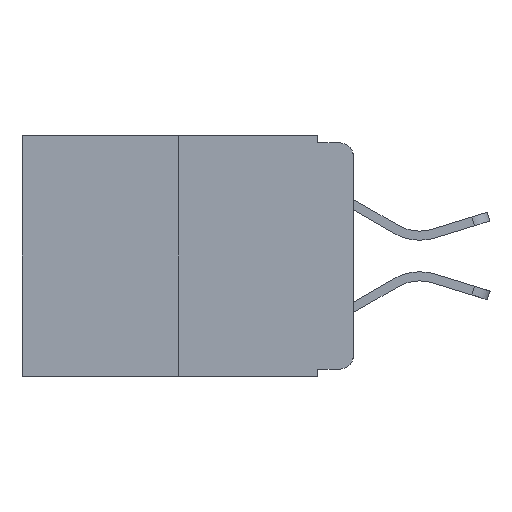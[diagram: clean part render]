
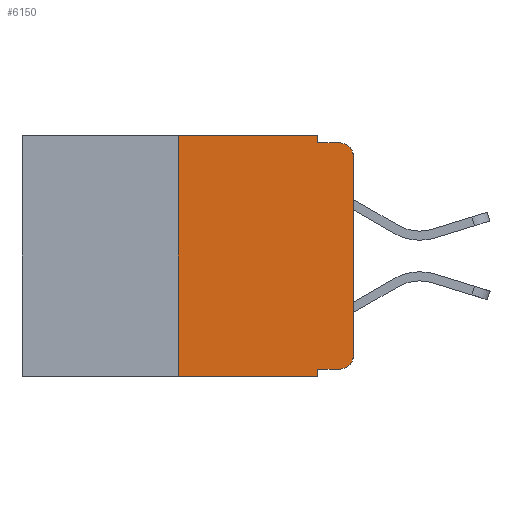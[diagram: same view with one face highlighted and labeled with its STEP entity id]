
A CAD part, left-side view. The second image highlights one B-rep face of the part: STEP entity #6150.
In plain terms, the highlighted planar face has unit normal (-1, 0, 0).
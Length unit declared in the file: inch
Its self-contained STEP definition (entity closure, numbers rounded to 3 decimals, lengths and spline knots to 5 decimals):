
#43 = CARTESIAN_POINT ( 'NONE',  ( 0., 0.02, -0.333 ) ) ;
#276 = AXIS2_PLACEMENT_3D ( 'NONE', #3128, #4411, #10474 ) ;
#378 = CARTESIAN_POINT ( 'NONE',  ( 0., 0.051, -0.333 ) ) ;
#526 = ORIENTED_EDGE ( 'NONE', *, *, #14124, .F. ) ;
#619 = DIRECTION ( 'NONE',  ( 0., 0., -1. ) ) ;
#1022 = ORIENTED_EDGE ( 'NONE', *, *, #7810, .T. ) ;
#1170 = VERTEX_POINT ( 'NONE', #5011 ) ;
#1910 = CARTESIAN_POINT ( 'NONE',  ( 0., 0.473, 0. ) ) ;
#2029 = EDGE_CURVE ( 'NONE', #13084, #7139, #14007, .T. ) ;
#2135 = ORIENTED_EDGE ( 'NONE', *, *, #12622, .F. ) ;
#2182 = ORIENTED_EDGE ( 'NONE', *, *, #7013, .T. ) ;
#2329 = VECTOR ( 'NONE', #5635, 39.37008 ) ;
#2383 = CARTESIAN_POINT ( 'NONE',  ( 0., 0.02, -0.03 ) ) ;
#2386 = LINE ( 'NONE', #9599, #8505 ) ;
#2451 = CARTESIAN_POINT ( 'NONE',  ( 0., 0.25, 0. ) ) ;
#2892 = VECTOR ( 'NONE', #12901, 39.37008 ) ;
#3107 = PLANE ( 'NONE',  #15008 ) ;
#3128 = CARTESIAN_POINT ( 'NONE',  ( 0., 0.02, -0.313 ) ) ;
#3246 = EDGE_CURVE ( 'NONE', #14308, #9445, #15822, .T. ) ;
#3332 = CIRCLE ( 'NONE', #16323, 0.02 ) ;
#3371 = CARTESIAN_POINT ( 'NONE',  ( 0., 0.25, -0.343 ) ) ;
#3635 = DIRECTION ( 'NONE',  ( 0., -1., 0. ) ) ;
#3846 = ORIENTED_EDGE ( 'NONE', *, *, #3246, .T. ) ;
#4153 = EDGE_CURVE ( 'NONE', #1170, #8397, #12977, .T. ) ;
#4252 = LINE ( 'NONE', #8271, #10768 ) ;
#4361 = CARTESIAN_POINT ( 'NONE',  ( 0., 0.473, -0.343 ) ) ;
#4411 = DIRECTION ( 'NONE',  ( -1., 0., 0. ) ) ;
#4662 = ORIENTED_EDGE ( 'NONE', *, *, #4153, .T. ) ;
#4852 = CARTESIAN_POINT ( 'NONE',  ( 0., 0.051, -0.01 ) ) ;
#5011 = CARTESIAN_POINT ( 'NONE',  ( 0., 0., -0.313 ) ) ;
#5635 = DIRECTION ( 'NONE',  ( 0., -1., 0. ) ) ;
#6150 = ADVANCED_FACE ( 'NONE', ( #14501 ), #3107, .F. ) ;
#6597 = VERTEX_POINT ( 'NONE', #2451 ) ;
#6792 = DIRECTION ( 'NONE',  ( 0., -1., 0. ) ) ;
#7013 = EDGE_CURVE ( 'NONE', #16116, #1170, #11058, .T. ) ;
#7139 = VERTEX_POINT ( 'NONE', #14568 ) ;
#7280 = EDGE_CURVE ( 'NONE', #8397, #7139, #3332, .T. ) ;
#7810 = EDGE_CURVE ( 'NONE', #12369, #16116, #14574, .T. ) ;
#7844 = VECTOR ( 'NONE', #10904, 39.37008 ) ;
#7974 = CARTESIAN_POINT ( 'NONE',  ( 0., 0.051, -0.343 ) ) ;
#8186 = DIRECTION ( 'NONE',  ( 1., 0., 0. ) ) ;
#8271 = CARTESIAN_POINT ( 'NONE',  ( 0., 0.051, 0. ) ) ;
#8397 = VERTEX_POINT ( 'NONE', #15776 ) ;
#8505 = VECTOR ( 'NONE', #13244, 39.37008 ) ;
#8633 = CARTESIAN_POINT ( 'NONE',  ( 0., 0.051, 0. ) ) ;
#8984 = CARTESIAN_POINT ( 'NONE',  ( 0., 0., 0. ) ) ;
#9010 = EDGE_LOOP ( 'NONE', ( #4662, #9664, #12788, #526, #15901, #13563, #3846, #2135, #1022, #2182 ) ) ;
#9445 = VERTEX_POINT ( 'NONE', #7974 ) ;
#9599 = CARTESIAN_POINT ( 'NONE',  ( 0., 0.25, 0. ) ) ;
#9664 = ORIENTED_EDGE ( 'NONE', *, *, #7280, .T. ) ;
#10061 = VECTOR ( 'NONE', #3635, 39.37008 ) ;
#10316 = LINE ( 'NONE', #1910, #13695 ) ;
#10474 = DIRECTION ( 'NONE',  ( 0., 0., -1. ) ) ;
#10639 = EDGE_CURVE ( 'NONE', #6597, #10917, #10316, .T. ) ;
#10768 = VECTOR ( 'NONE', #11885, 39.37008 ) ;
#10904 = DIRECTION ( 'NONE',  ( 0., -1., 0. ) ) ;
#10917 = VERTEX_POINT ( 'NONE', #8633 ) ;
#11058 = CIRCLE ( 'NONE', #276, 0.02 ) ;
#11671 = LINE ( 'NONE', #15241, #12075 ) ;
#11885 = DIRECTION ( 'NONE',  ( 0., 0., -1. ) ) ;
#12075 = VECTOR ( 'NONE', #15297, 39.37008 ) ;
#12369 = VERTEX_POINT ( 'NONE', #378 ) ;
#12622 = EDGE_CURVE ( 'NONE', #12369, #9445, #11671, .T. ) ;
#12788 = ORIENTED_EDGE ( 'NONE', *, *, #2029, .F. ) ;
#12901 = DIRECTION ( 'NONE',  ( 0., 0., 1. ) ) ;
#12977 = LINE ( 'NONE', #8984, #2892 ) ;
#13084 = VERTEX_POINT ( 'NONE', #14732 ) ;
#13244 = DIRECTION ( 'NONE',  ( 0., 0., 1. ) ) ;
#13563 = ORIENTED_EDGE ( 'NONE', *, *, #15840, .F. ) ;
#13624 = DIRECTION ( 'NONE',  ( 0., 0., -1. ) ) ;
#13695 = VECTOR ( 'NONE', #6792, 39.37008 ) ;
#14007 = LINE ( 'NONE', #4852, #10061 ) ;
#14124 = EDGE_CURVE ( 'NONE', #10917, #13084, #4252, .T. ) ;
#14308 = VERTEX_POINT ( 'NONE', #3371 ) ;
#14501 = FACE_OUTER_BOUND ( 'NONE', #9010, .T. ) ;
#14568 = CARTESIAN_POINT ( 'NONE',  ( 0., 0.02, -0.01 ) ) ;
#14574 = LINE ( 'NONE', #16072, #7844 ) ;
#14732 = CARTESIAN_POINT ( 'NONE',  ( 0., 0.051, -0.01 ) ) ;
#15008 = AXIS2_PLACEMENT_3D ( 'NONE', #15797, #8186, #619 ) ;
#15241 = CARTESIAN_POINT ( 'NONE',  ( 0., 0.051, 0. ) ) ;
#15297 = DIRECTION ( 'NONE',  ( 0., 0., -1. ) ) ;
#15776 = CARTESIAN_POINT ( 'NONE',  ( 0., 0., -0.03 ) ) ;
#15797 = CARTESIAN_POINT ( 'NONE',  ( 0., 0.473, 0. ) ) ;
#15822 = LINE ( 'NONE', #4361, #2329 ) ;
#15840 = EDGE_CURVE ( 'NONE', #14308, #6597, #2386, .T. ) ;
#15901 = ORIENTED_EDGE ( 'NONE', *, *, #10639, .F. ) ;
#16072 = CARTESIAN_POINT ( 'NONE',  ( 0., 0.051, -0.333 ) ) ;
#16116 = VERTEX_POINT ( 'NONE', #43 ) ;
#16244 = DIRECTION ( 'NONE',  ( -1., 0., 0. ) ) ;
#16323 = AXIS2_PLACEMENT_3D ( 'NONE', #2383, #16244, #13624 ) ;
